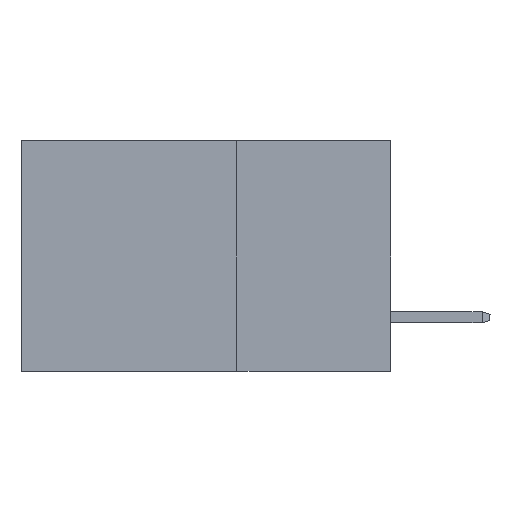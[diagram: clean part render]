
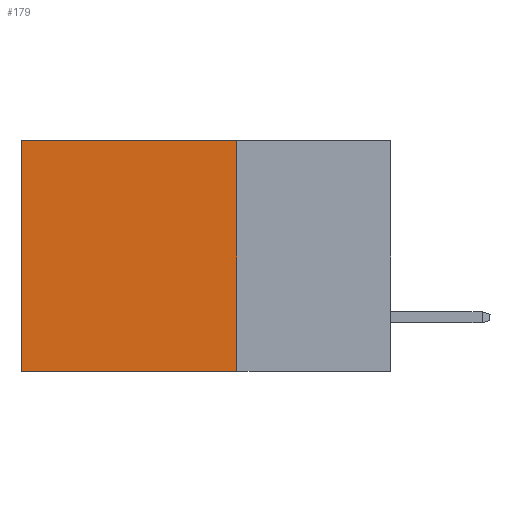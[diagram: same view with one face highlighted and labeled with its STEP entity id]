
A CAD part, left-side view. The second image highlights one B-rep face of the part: STEP entity #179.
In plain terms, the highlighted planar face has unit normal (-1, 0, 0).
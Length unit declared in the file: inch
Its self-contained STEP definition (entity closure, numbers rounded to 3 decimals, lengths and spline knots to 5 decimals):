
#82 = LINE ( 'NONE', #9167, #3130 ) ;
#179 = ADVANCED_FACE ( 'NONE', ( #7941 ), #4254, .F. ) ;
#277 = CARTESIAN_POINT ( 'NONE',  ( 0.2875, 0.6, 0. ) ) ;
#792 = VERTEX_POINT ( 'NONE', #277 ) ;
#1137 = VECTOR ( 'NONE', #8835, 39.37008 ) ;
#1225 = EDGE_LOOP ( 'NONE', ( #6869, #5485, #6006, #3386 ) ) ;
#1328 = DIRECTION ( 'NONE',  ( 0., 0., -1. ) ) ;
#1428 = VERTEX_POINT ( 'NONE', #8649 ) ;
#1484 = CARTESIAN_POINT ( 'NONE',  ( 0.2875, 0.25, 0. ) ) ;
#1935 = CARTESIAN_POINT ( 'NONE',  ( 0.2875, 0.6, -0.375 ) ) ;
#2007 = CARTESIAN_POINT ( 'NONE',  ( 0.2875, 0.6, -0.375 ) ) ;
#2069 = DIRECTION ( 'NONE',  ( 0., 1., 0. ) ) ;
#2615 = DIRECTION ( 'NONE',  ( 0., 0., -1. ) ) ;
#3130 = VECTOR ( 'NONE', #2615, 39.37008 ) ;
#3386 = ORIENTED_EDGE ( 'NONE', *, *, #3613, .T. ) ;
#3424 = VERTEX_POINT ( 'NONE', #3530 ) ;
#3530 = CARTESIAN_POINT ( 'NONE',  ( 0.2875, 0.25, 0. ) ) ;
#3613 = EDGE_CURVE ( 'NONE', #3424, #792, #7495, .T. ) ;
#4254 = PLANE ( 'NONE',  #4555 ) ;
#4555 = AXIS2_PLACEMENT_3D ( 'NONE', #7871, #9429, #1328 ) ;
#5485 = ORIENTED_EDGE ( 'NONE', *, *, #7460, .F. ) ;
#5819 = CARTESIAN_POINT ( 'NONE',  ( 0.2875, 0.25, -0.375 ) ) ;
#5936 = EDGE_CURVE ( 'NONE', #3424, #1428, #82, .T. ) ;
#6006 = ORIENTED_EDGE ( 'NONE', *, *, #5936, .F. ) ;
#6869 = ORIENTED_EDGE ( 'NONE', *, *, #7396, .T. ) ;
#7115 = DIRECTION ( 'NONE',  ( 0., 0., -1. ) ) ;
#7396 = EDGE_CURVE ( 'NONE', #792, #8732, #7852, .T. ) ;
#7460 = EDGE_CURVE ( 'NONE', #1428, #8732, #9104, .T. ) ;
#7495 = LINE ( 'NONE', #1484, #1137 ) ;
#7623 = VECTOR ( 'NONE', #7115, 39.37008 ) ;
#7852 = LINE ( 'NONE', #1935, #7623 ) ;
#7871 = CARTESIAN_POINT ( 'NONE',  ( 0.2875, 0.25, -0.375 ) ) ;
#7941 = FACE_OUTER_BOUND ( 'NONE', #1225, .T. ) ;
#8649 = CARTESIAN_POINT ( 'NONE',  ( 0.2875, 0.25, -0.375 ) ) ;
#8732 = VERTEX_POINT ( 'NONE', #2007 ) ;
#8771 = VECTOR ( 'NONE', #2069, 39.37008 ) ;
#8835 = DIRECTION ( 'NONE',  ( 0., 1., 0. ) ) ;
#9104 = LINE ( 'NONE', #5819, #8771 ) ;
#9167 = CARTESIAN_POINT ( 'NONE',  ( 0.2875, 0.25, -0.375 ) ) ;
#9429 = DIRECTION ( 'NONE',  ( 1., 0., 0. ) ) ;
